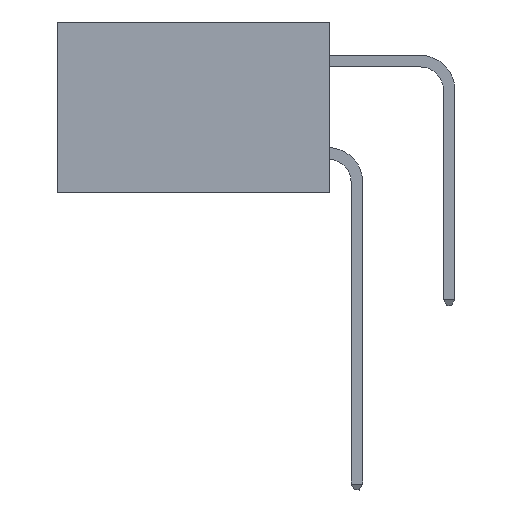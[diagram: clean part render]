
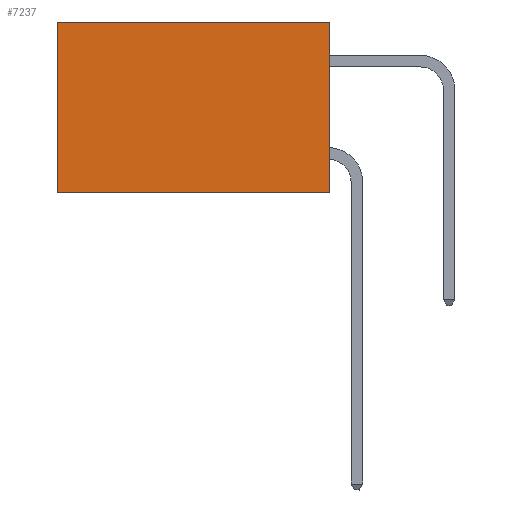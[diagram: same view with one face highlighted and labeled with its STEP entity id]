
A CAD part, left-side view. The second image highlights one B-rep face of the part: STEP entity #7237.
In plain terms, the highlighted planar face has unit normal (-1, 0, 0).
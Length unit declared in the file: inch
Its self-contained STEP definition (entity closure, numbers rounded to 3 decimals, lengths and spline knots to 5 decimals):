
#663 = DIRECTION ( 'NONE',  ( 0., 1., 0. ) ) ;
#1727 = ORIENTED_EDGE ( 'NONE', *, *, #22784, .F. ) ;
#1819 = LINE ( 'NONE', #4766, #16940 ) ;
#3542 = ORIENTED_EDGE ( 'NONE', *, *, #20939, .T. ) ;
#4584 = VERTEX_POINT ( 'NONE', #20455 ) ;
#4766 = CARTESIAN_POINT ( 'NONE',  ( 0.277, 0.59, -0.37 ) ) ;
#5138 = LINE ( 'NONE', #7549, #15439 ) ;
#6243 = CARTESIAN_POINT ( 'NONE',  ( 0.277, 0., -0.37 ) ) ;
#6603 = CARTESIAN_POINT ( 'NONE',  ( 0.277, 0.59, 0. ) ) ;
#7237 = ADVANCED_FACE ( 'NONE', ( #8110 ), #18490, .F. ) ;
#7549 = CARTESIAN_POINT ( 'NONE',  ( 0.277, 0., -0.37 ) ) ;
#8110 = FACE_OUTER_BOUND ( 'NONE', #10853, .T. ) ;
#10406 = DIRECTION ( 'NONE',  ( 1., 0., 0. ) ) ;
#10645 = LINE ( 'NONE', #18905, #15452 ) ;
#10656 = VERTEX_POINT ( 'NONE', #20969 ) ;
#10853 = EDGE_LOOP ( 'NONE', ( #3542, #1727, #18471, #20276 ) ) ;
#10988 = CARTESIAN_POINT ( 'NONE',  ( 0.277, 0., 0. ) ) ;
#14524 = VERTEX_POINT ( 'NONE', #20238 ) ;
#15439 = VECTOR ( 'NONE', #19743, 39.37008 ) ;
#15452 = VECTOR ( 'NONE', #20922, 39.37008 ) ;
#16940 = VECTOR ( 'NONE', #21091, 39.37008 ) ;
#18471 = ORIENTED_EDGE ( 'NONE', *, *, #19902, .F. ) ;
#18490 = PLANE ( 'NONE',  #19213 ) ;
#18872 = VERTEX_POINT ( 'NONE', #6603 ) ;
#18905 = CARTESIAN_POINT ( 'NONE',  ( 0.277, 0., -0.37 ) ) ;
#19133 = LINE ( 'NONE', #10988, #23841 ) ;
#19213 = AXIS2_PLACEMENT_3D ( 'NONE', #6243, #10406, #24571 ) ;
#19743 = DIRECTION ( 'NONE',  ( 0., 0., -1. ) ) ;
#19902 = EDGE_CURVE ( 'NONE', #4584, #10656, #5138, .T. ) ;
#20238 = CARTESIAN_POINT ( 'NONE',  ( 0.277, 0.59, -0.37 ) ) ;
#20276 = ORIENTED_EDGE ( 'NONE', *, *, #25106, .T. ) ;
#20455 = CARTESIAN_POINT ( 'NONE',  ( 0.277, 0., 0. ) ) ;
#20922 = DIRECTION ( 'NONE',  ( 0., 1., 0. ) ) ;
#20939 = EDGE_CURVE ( 'NONE', #18872, #14524, #1819, .T. ) ;
#20969 = CARTESIAN_POINT ( 'NONE',  ( 0.277, 0., -0.37 ) ) ;
#21091 = DIRECTION ( 'NONE',  ( 0., 0., -1. ) ) ;
#22784 = EDGE_CURVE ( 'NONE', #10656, #14524, #10645, .T. ) ;
#23841 = VECTOR ( 'NONE', #663, 39.37008 ) ;
#24571 = DIRECTION ( 'NONE',  ( 0., 0., -1. ) ) ;
#25106 = EDGE_CURVE ( 'NONE', #4584, #18872, #19133, .T. ) ;
